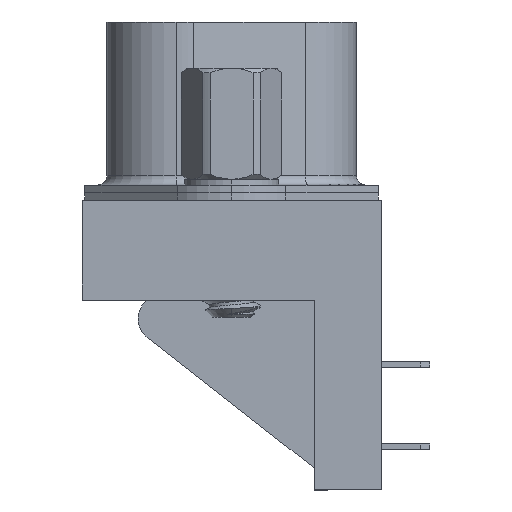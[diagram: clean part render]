
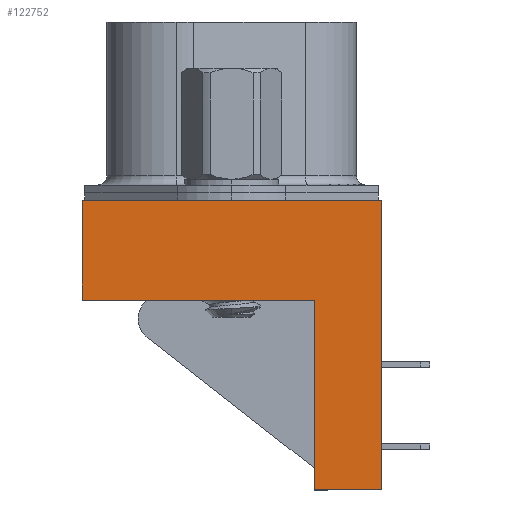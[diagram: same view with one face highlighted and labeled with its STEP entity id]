
A CAD part, left-side view. The second image highlights one B-rep face of the part: STEP entity #122752.
In plain terms, the highlighted planar face has unit normal (-1, 0, 0).
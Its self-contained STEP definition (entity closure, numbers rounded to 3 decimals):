
#827 = EDGE_CURVE ( 'NONE', #127609, #111782, #834, .T. ) ;
#834 = LINE ( 'NONE', #114127, #1677 ) ;
#1677 = VECTOR ( 'NONE', #170898, 1000. ) ;
#5661 = DIRECTION ( 'NONE',  ( 0., 1., 0. ) ) ;
#10942 = CARTESIAN_POINT ( 'NONE',  ( -4.125, -4.3, -5.2 ) ) ;
#12525 = DIRECTION ( 'NONE',  ( 0., 0., 1. ) ) ;
#24795 = CARTESIAN_POINT ( 'NONE',  ( -4.125, 7.8, -5.2 ) ) ;
#25423 = EDGE_CURVE ( 'NONE', #149594, #138996, #103600, .T. ) ;
#29048 = VECTOR ( 'NONE', #5661, 1000. ) ;
#31561 = EDGE_LOOP ( 'NONE', ( #138675, #71033, #78770, #173205, #168869, #148808 ) ) ;
#45126 = VERTEX_POINT ( 'NONE', #97561 ) ;
#62719 = LINE ( 'NONE', #119386, #84444 ) ;
#67687 = VECTOR ( 'NONE', #12525, 1000. ) ;
#68285 = LINE ( 'NONE', #181706, #67687 ) ;
#68406 = CARTESIAN_POINT ( 'NONE',  ( -4.125, 7.8, -15.1 ) ) ;
#68861 = CARTESIAN_POINT ( 'NONE',  ( -4.125, -7.8, 0. ) ) ;
#70230 = LINE ( 'NONE', #68406, #71758 ) ;
#71033 = ORIENTED_EDGE ( 'NONE', *, *, #827, .F. ) ;
#71758 = VECTOR ( 'NONE', #97178, 1000. ) ;
#78770 = ORIENTED_EDGE ( 'NONE', *, *, #181120, .T. ) ;
#80634 = VECTOR ( 'NONE', #130562, 1000. ) ;
#84444 = VECTOR ( 'NONE', #176144, 1000. ) ;
#87489 = DIRECTION ( 'NONE',  ( 0., -1., 0. ) ) ;
#96204 = EDGE_CURVE ( 'NONE', #111782, #136826, #133865, .T. ) ;
#97178 = DIRECTION ( 'NONE',  ( 0., -1., 0. ) ) ;
#97561 = CARTESIAN_POINT ( 'NONE',  ( -4.125, -7.8, -15.1 ) ) ;
#102339 = PLANE ( 'NONE',  #166160 ) ;
#103600 = LINE ( 'NONE', #145438, #80634 ) ;
#111782 = VERTEX_POINT ( 'NONE', #10942 ) ;
#114127 = CARTESIAN_POINT ( 'NONE',  ( -4.125, -4.3, -15.1 ) ) ;
#119386 = CARTESIAN_POINT ( 'NONE',  ( -4.125, -7.8, -15.1 ) ) ;
#121072 = EDGE_CURVE ( 'NONE', #136826, #149594, #68285, .T. ) ;
#122752 = ADVANCED_FACE ( 'NONE', ( #143274 ), #102339, .T. ) ;
#127609 = VERTEX_POINT ( 'NONE', #135389 ) ;
#130562 = DIRECTION ( 'NONE',  ( 0., -1., 0. ) ) ;
#133865 = LINE ( 'NONE', #24795, #29048 ) ;
#135389 = CARTESIAN_POINT ( 'NONE',  ( -4.125, -4.3, -15.1 ) ) ;
#136826 = VERTEX_POINT ( 'NONE', #183266 ) ;
#138675 = ORIENTED_EDGE ( 'NONE', *, *, #96204, .F. ) ;
#138996 = VERTEX_POINT ( 'NONE', #68861 ) ;
#139563 = EDGE_CURVE ( 'NONE', #45126, #138996, #62719, .T. ) ;
#141461 = DIRECTION ( 'NONE',  ( -1., 0., 0. ) ) ;
#143274 = FACE_OUTER_BOUND ( 'NONE', #31561, .T. ) ;
#145438 = CARTESIAN_POINT ( 'NONE',  ( -4.125, 7.8, 0. ) ) ;
#148808 = ORIENTED_EDGE ( 'NONE', *, *, #121072, .F. ) ;
#149594 = VERTEX_POINT ( 'NONE', #173370 ) ;
#157250 = CARTESIAN_POINT ( 'NONE',  ( -4.125, 7.8, -15.1 ) ) ;
#166160 = AXIS2_PLACEMENT_3D ( 'NONE', #157250, #141461, #87489 ) ;
#168869 = ORIENTED_EDGE ( 'NONE', *, *, #25423, .F. ) ;
#170898 = DIRECTION ( 'NONE',  ( 0., 0., 1. ) ) ;
#173205 = ORIENTED_EDGE ( 'NONE', *, *, #139563, .T. ) ;
#173370 = CARTESIAN_POINT ( 'NONE',  ( -4.125, 7.8, 0. ) ) ;
#176144 = DIRECTION ( 'NONE',  ( 0., 0., 1. ) ) ;
#181120 = EDGE_CURVE ( 'NONE', #127609, #45126, #70230, .T. ) ;
#181706 = CARTESIAN_POINT ( 'NONE',  ( -4.125, 7.8, -15.1 ) ) ;
#183266 = CARTESIAN_POINT ( 'NONE',  ( -4.125, 7.8, -5.2 ) ) ;
